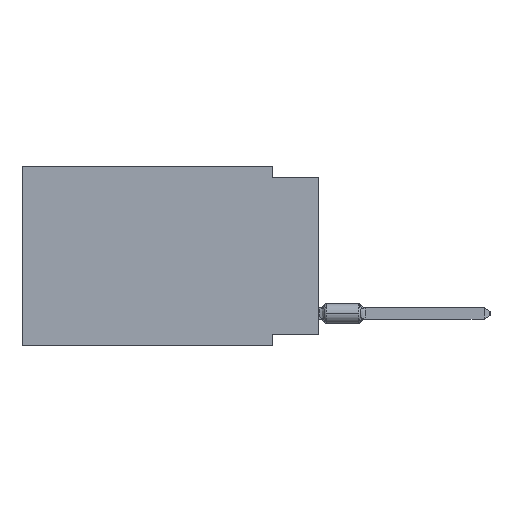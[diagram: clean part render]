
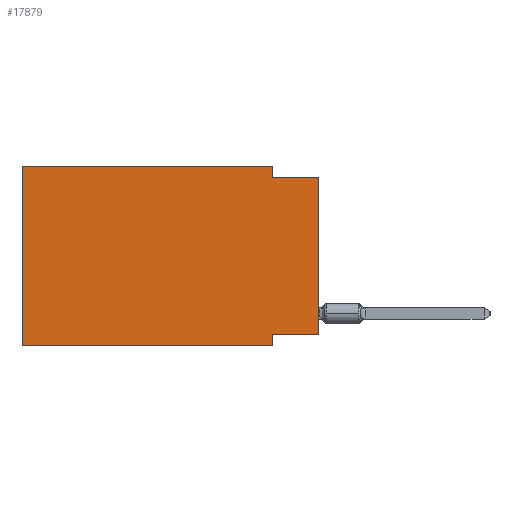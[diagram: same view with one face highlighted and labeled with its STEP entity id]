
A CAD part, left-side view. The second image highlights one B-rep face of the part: STEP entity #17879.
In plain terms, the highlighted planar face has unit normal (-1, 0, 0).
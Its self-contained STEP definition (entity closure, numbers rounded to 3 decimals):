
#232 = CARTESIAN_POINT ( 'NONE',  ( 0., 16.383, 0. ) ) ;
#906 = CARTESIAN_POINT ( 'NONE',  ( 0., 0., -0.635 ) ) ;
#3380 = VERTEX_POINT ( 'NONE', #60415 ) ;
#4444 = EDGE_CURVE ( 'NONE', #12685, #45461, #65059, .T. ) ;
#5075 = LINE ( 'NONE', #26077, #31654 ) ;
#5117 = DIRECTION ( 'NONE',  ( 0., 0., -1. ) ) ;
#5682 = CARTESIAN_POINT ( 'NONE',  ( 0., 16.383, 0. ) ) ;
#6031 = EDGE_CURVE ( 'NONE', #49969, #12685, #29540, .T. ) ;
#7653 = EDGE_LOOP ( 'NONE', ( #35189, #27260, #52285, #22406, #66609, #15332, #41152, #54536 ) ) ;
#8107 = LINE ( 'NONE', #35103, #63179 ) ;
#8720 = VECTOR ( 'NONE', #19224, 1000. ) ;
#8792 = EDGE_CURVE ( 'NONE', #45461, #66796, #8107, .T. ) ;
#8800 = PLANE ( 'NONE',  #40315 ) ;
#8958 = EDGE_CURVE ( 'NONE', #3380, #54184, #13784, .T. ) ;
#9729 = LINE ( 'NONE', #69451, #10769 ) ;
#10769 = VECTOR ( 'NONE', #48469, 1000. ) ;
#12685 = VERTEX_POINT ( 'NONE', #232 ) ;
#13784 = LINE ( 'NONE', #67928, #8720 ) ;
#15332 = ORIENTED_EDGE ( 'NONE', *, *, #36084, .T. ) ;
#16134 = VERTEX_POINT ( 'NONE', #59433 ) ;
#16684 = CARTESIAN_POINT ( 'NONE',  ( 0., 16.383, -9.906 ) ) ;
#17879 = ADVANCED_FACE ( 'NONE', ( #25162 ), #8800, .F. ) ;
#19224 = DIRECTION ( 'NONE',  ( 0., 1., 0. ) ) ;
#20151 = DIRECTION ( 'NONE',  ( 0., 0., -1. ) ) ;
#20158 = DIRECTION ( 'NONE',  ( 0., 0., -1. ) ) ;
#22406 = ORIENTED_EDGE ( 'NONE', *, *, #4444, .F. ) ;
#25162 = FACE_OUTER_BOUND ( 'NONE', #7653, .T. ) ;
#26077 = CARTESIAN_POINT ( 'NONE',  ( 0., 16.383, -9.906 ) ) ;
#27260 = ORIENTED_EDGE ( 'NONE', *, *, #40460, .F. ) ;
#29540 = LINE ( 'NONE', #30945, #38622 ) ;
#30945 = CARTESIAN_POINT ( 'NONE',  ( 0., 16.383, 0. ) ) ;
#31158 = CARTESIAN_POINT ( 'NONE',  ( 0., 16.383, 0. ) ) ;
#31654 = VECTOR ( 'NONE', #69438, 1000. ) ;
#33000 = VECTOR ( 'NONE', #44628, 1000. ) ;
#33151 = VECTOR ( 'NONE', #5117, 1000. ) ;
#35103 = CARTESIAN_POINT ( 'NONE',  ( 0., 2.54, 0. ) ) ;
#35189 = ORIENTED_EDGE ( 'NONE', *, *, #66528, .T. ) ;
#35896 = DIRECTION ( 'NONE',  ( 0., 0., 1. ) ) ;
#36084 = EDGE_CURVE ( 'NONE', #49969, #16134, #5075, .T. ) ;
#36755 = LINE ( 'NONE', #37108, #33151 ) ;
#36908 = CARTESIAN_POINT ( 'NONE',  ( 0., 2.54, -0.635 ) ) ;
#37108 = CARTESIAN_POINT ( 'NONE',  ( 0., 2.54, -9.906 ) ) ;
#38622 = VECTOR ( 'NONE', #35896, 1000. ) ;
#40315 = AXIS2_PLACEMENT_3D ( 'NONE', #31158, #69546, #20151 ) ;
#40460 = EDGE_CURVE ( 'NONE', #66796, #65278, #44976, .T. ) ;
#41152 = ORIENTED_EDGE ( 'NONE', *, *, #41830, .F. ) ;
#41830 = EDGE_CURVE ( 'NONE', #54184, #16134, #36755, .T. ) ;
#43366 = DIRECTION ( 'NONE',  ( 0., -1., 0. ) ) ;
#44628 = DIRECTION ( 'NONE',  ( 0., -1., 0. ) ) ;
#44976 = LINE ( 'NONE', #906, #33000 ) ;
#45461 = VERTEX_POINT ( 'NONE', #45892 ) ;
#45892 = CARTESIAN_POINT ( 'NONE',  ( 0., 2.54, 0. ) ) ;
#48469 = DIRECTION ( 'NONE',  ( 0., 0., 1. ) ) ;
#49892 = VECTOR ( 'NONE', #43366, 1000. ) ;
#49969 = VERTEX_POINT ( 'NONE', #16684 ) ;
#52285 = ORIENTED_EDGE ( 'NONE', *, *, #8792, .F. ) ;
#53548 = CARTESIAN_POINT ( 'NONE',  ( 0., 2.54, -9.271 ) ) ;
#54089 = CARTESIAN_POINT ( 'NONE',  ( 0., 0., -0.635 ) ) ;
#54184 = VERTEX_POINT ( 'NONE', #53548 ) ;
#54536 = ORIENTED_EDGE ( 'NONE', *, *, #8958, .F. ) ;
#59433 = CARTESIAN_POINT ( 'NONE',  ( 0., 2.54, -9.906 ) ) ;
#60415 = CARTESIAN_POINT ( 'NONE',  ( 0., 0., -9.271 ) ) ;
#63179 = VECTOR ( 'NONE', #20158, 1000. ) ;
#65059 = LINE ( 'NONE', #5682, #49892 ) ;
#65278 = VERTEX_POINT ( 'NONE', #54089 ) ;
#66528 = EDGE_CURVE ( 'NONE', #3380, #65278, #9729, .T. ) ;
#66609 = ORIENTED_EDGE ( 'NONE', *, *, #6031, .F. ) ;
#66796 = VERTEX_POINT ( 'NONE', #36908 ) ;
#67928 = CARTESIAN_POINT ( 'NONE',  ( 0., 0., -9.271 ) ) ;
#69438 = DIRECTION ( 'NONE',  ( 0., -1., 0. ) ) ;
#69451 = CARTESIAN_POINT ( 'NONE',  ( 0., 0., 0. ) ) ;
#69546 = DIRECTION ( 'NONE',  ( 1., 0., 0. ) ) ;
